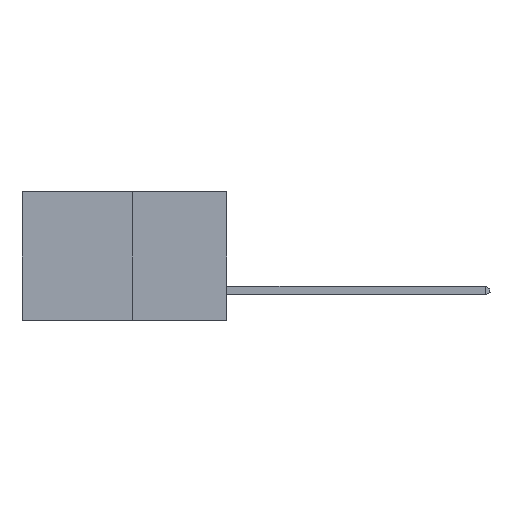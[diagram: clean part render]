
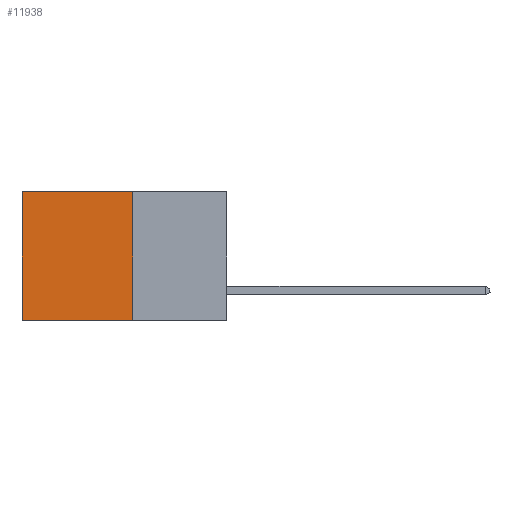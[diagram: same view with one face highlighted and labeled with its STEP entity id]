
A CAD part, left-side view. The second image highlights one B-rep face of the part: STEP entity #11938.
In plain terms, the highlighted planar face has unit normal (-1, 0, 0).
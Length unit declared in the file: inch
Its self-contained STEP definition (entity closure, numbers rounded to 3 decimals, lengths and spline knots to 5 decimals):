
#303 = EDGE_CURVE ( 'NONE', #28285, #7702, #3979, .T. ) ;
#1739 = DIRECTION ( 'NONE',  ( 0., 0., -1. ) ) ;
#2615 = CARTESIAN_POINT ( 'NONE',  ( 0.277, 0.27, 0. ) ) ;
#2722 = LINE ( 'NONE', #2615, #21796 ) ;
#3404 = CARTESIAN_POINT ( 'NONE',  ( 0.277, 0.27, 0. ) ) ;
#3463 = CARTESIAN_POINT ( 'NONE',  ( 0.277, 0.27, -0.37 ) ) ;
#3979 = LINE ( 'NONE', #3463, #14852 ) ;
#5298 = CARTESIAN_POINT ( 'NONE',  ( 0.277, 0.27, -0.37 ) ) ;
#6022 = CARTESIAN_POINT ( 'NONE',  ( 0.277, 0.59, -0.37 ) ) ;
#6209 = VECTOR ( 'NONE', #24725, 39.37008 ) ;
#6344 = AXIS2_PLACEMENT_3D ( 'NONE', #19069, #16635, #1739 ) ;
#7702 = VERTEX_POINT ( 'NONE', #6022 ) ;
#7780 = LINE ( 'NONE', #22207, #6209 ) ;
#8077 = ORIENTED_EDGE ( 'NONE', *, *, #12088, .T. ) ;
#8301 = VERTEX_POINT ( 'NONE', #3404 ) ;
#9838 = VECTOR ( 'NONE', #22896, 39.37008 ) ;
#11938 = ADVANCED_FACE ( 'NONE', ( #30780 ), #26585, .F. ) ;
#12088 = EDGE_CURVE ( 'NONE', #26369, #7702, #7780, .T. ) ;
#12234 = ORIENTED_EDGE ( 'NONE', *, *, #22586, .F. ) ;
#12568 = CARTESIAN_POINT ( 'NONE',  ( 0.277, 0.59, 0. ) ) ;
#14852 = VECTOR ( 'NONE', #27960, 39.37008 ) ;
#16635 = DIRECTION ( 'NONE',  ( 1., 0., 0. ) ) ;
#19069 = CARTESIAN_POINT ( 'NONE',  ( 0.277, 0.27, -0.37 ) ) ;
#20005 = DIRECTION ( 'NONE',  ( 0., 1., 0. ) ) ;
#20426 = EDGE_CURVE ( 'NONE', #8301, #26369, #2722, .T. ) ;
#20482 = CARTESIAN_POINT ( 'NONE',  ( 0.277, 0.27, -0.37 ) ) ;
#21796 = VECTOR ( 'NONE', #20005, 39.37008 ) ;
#22207 = CARTESIAN_POINT ( 'NONE',  ( 0.277, 0.59, -0.37 ) ) ;
#22357 = EDGE_LOOP ( 'NONE', ( #8077, #31105, #12234, #25350 ) ) ;
#22586 = EDGE_CURVE ( 'NONE', #8301, #28285, #23904, .T. ) ;
#22896 = DIRECTION ( 'NONE',  ( 0., 0., -1. ) ) ;
#23904 = LINE ( 'NONE', #20482, #9838 ) ;
#24725 = DIRECTION ( 'NONE',  ( 0., 0., -1. ) ) ;
#25350 = ORIENTED_EDGE ( 'NONE', *, *, #20426, .T. ) ;
#26369 = VERTEX_POINT ( 'NONE', #12568 ) ;
#26585 = PLANE ( 'NONE',  #6344 ) ;
#27960 = DIRECTION ( 'NONE',  ( 0., 1., 0. ) ) ;
#28285 = VERTEX_POINT ( 'NONE', #5298 ) ;
#30780 = FACE_OUTER_BOUND ( 'NONE', #22357, .T. ) ;
#31105 = ORIENTED_EDGE ( 'NONE', *, *, #303, .F. ) ;
